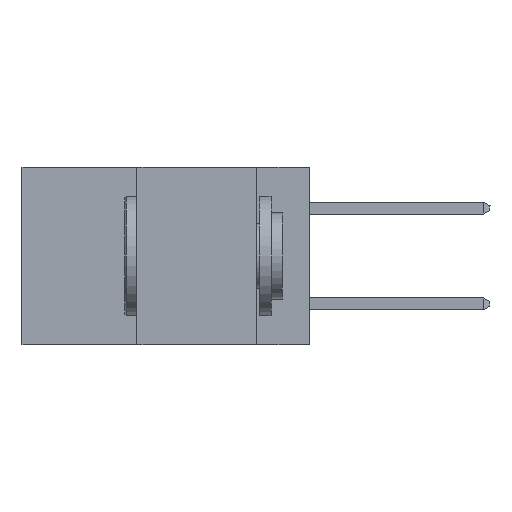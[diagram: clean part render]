
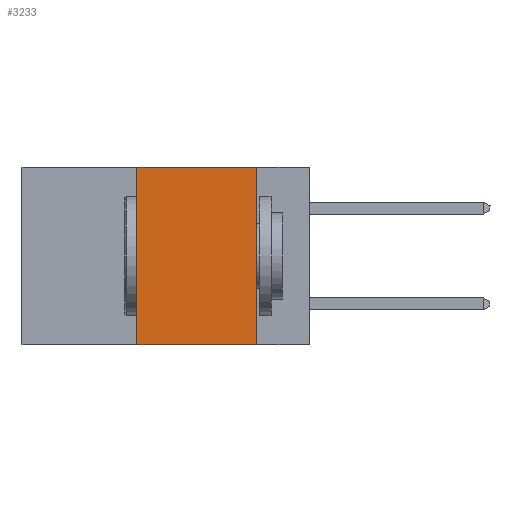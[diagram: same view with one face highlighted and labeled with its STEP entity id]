
A CAD part, left-side view. The second image highlights one B-rep face of the part: STEP entity #3233.
In plain terms, the highlighted planar face has unit normal (-1, 0, 0).
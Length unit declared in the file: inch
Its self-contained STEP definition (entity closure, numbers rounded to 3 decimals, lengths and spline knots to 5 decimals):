
#317 = ORIENTED_EDGE ( 'NONE', *, *, #8364, .F. ) ;
#1836 = DIRECTION ( 'NONE',  ( 0., 0., -1. ) ) ;
#2752 = VERTEX_POINT ( 'NONE', #38288 ) ;
#3233 = ADVANCED_FACE ( 'NONE', ( #26566 ), #28792, .F. ) ;
#3361 = VERTEX_POINT ( 'NONE', #11610 ) ;
#3496 = ORIENTED_EDGE ( 'NONE', *, *, #18805, .F. ) ;
#4115 = VECTOR ( 'NONE', #28158, 39.37008 ) ;
#7589 = DIRECTION ( 'NONE',  ( 0., 0., 1. ) ) ;
#7660 = DIRECTION ( 'NONE',  ( 0., -1., 0. ) ) ;
#8141 = VECTOR ( 'NONE', #7589, 39.37008 ) ;
#8364 = EDGE_CURVE ( 'NONE', #23474, #3361, #28136, .T. ) ;
#11363 = CARTESIAN_POINT ( 'NONE',  ( 0., 0.36, 0. ) ) ;
#11610 = CARTESIAN_POINT ( 'NONE',  ( 0., 0.11, -0.37 ) ) ;
#12100 = EDGE_CURVE ( 'NONE', #2752, #31093, #21307, .T. ) ;
#13217 = CARTESIAN_POINT ( 'NONE',  ( 0., 0.11, 0. ) ) ;
#15392 = EDGE_CURVE ( 'NONE', #2752, #3361, #25219, .T. ) ;
#18770 = CARTESIAN_POINT ( 'NONE',  ( 0., 0.11, 0. ) ) ;
#18805 = EDGE_CURVE ( 'NONE', #31093, #23474, #22623, .T. ) ;
#19819 = ORIENTED_EDGE ( 'NONE', *, *, #12100, .F. ) ;
#20033 = DIRECTION ( 'NONE',  ( 1., 0., 0. ) ) ;
#21307 = LINE ( 'NONE', #22579, #8141 ) ;
#22579 = CARTESIAN_POINT ( 'NONE',  ( 0., 0.36, 0. ) ) ;
#22623 = LINE ( 'NONE', #38594, #30622 ) ;
#22649 = CARTESIAN_POINT ( 'NONE',  ( 0., 0.6, -0.37 ) ) ;
#23474 = VERTEX_POINT ( 'NONE', #18770 ) ;
#25219 = LINE ( 'NONE', #22649, #38275 ) ;
#26566 = FACE_OUTER_BOUND ( 'NONE', #38896, .T. ) ;
#26776 = DIRECTION ( 'NONE',  ( 0., -1., 0. ) ) ;
#28136 = LINE ( 'NONE', #13217, #4115 ) ;
#28158 = DIRECTION ( 'NONE',  ( 0., 0., -1. ) ) ;
#28792 = PLANE ( 'NONE',  #36216 ) ;
#30622 = VECTOR ( 'NONE', #26776, 39.37008 ) ;
#31093 = VERTEX_POINT ( 'NONE', #11363 ) ;
#36216 = AXIS2_PLACEMENT_3D ( 'NONE', #37899, #20033, #1836 ) ;
#37899 = CARTESIAN_POINT ( 'NONE',  ( 0., 0.6, 0. ) ) ;
#38275 = VECTOR ( 'NONE', #7660, 39.37008 ) ;
#38288 = CARTESIAN_POINT ( 'NONE',  ( 0., 0.36, -0.37 ) ) ;
#38594 = CARTESIAN_POINT ( 'NONE',  ( 0., 0.6, 0. ) ) ;
#38896 = EDGE_LOOP ( 'NONE', ( #317, #3496, #19819, #38910 ) ) ;
#38910 = ORIENTED_EDGE ( 'NONE', *, *, #15392, .T. ) ;
